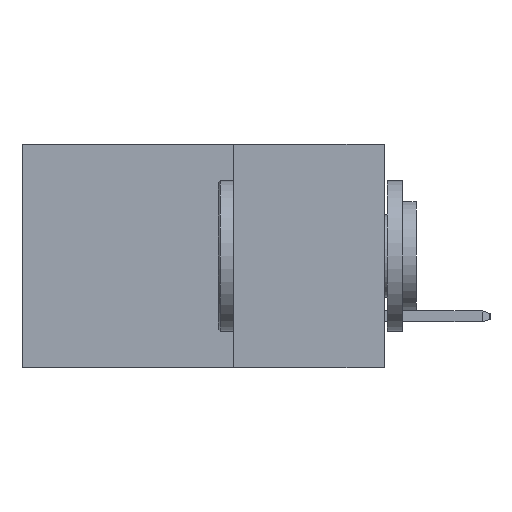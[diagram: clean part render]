
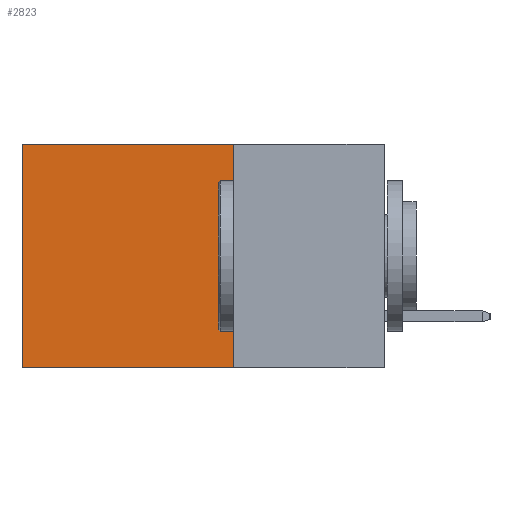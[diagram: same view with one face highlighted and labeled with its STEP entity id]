
A CAD part, left-side view. The second image highlights one B-rep face of the part: STEP entity #2823.
In plain terms, the highlighted planar face has unit normal (-1, 0, 0).
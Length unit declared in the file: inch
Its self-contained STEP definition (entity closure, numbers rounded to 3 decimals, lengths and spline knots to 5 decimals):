
#267 = ORIENTED_EDGE ( 'NONE', *, *, #7602, .F. ) ;
#420 = DIRECTION ( 'NONE',  ( 0., 1., 0. ) ) ;
#733 = VERTEX_POINT ( 'NONE', #10349 ) ;
#1479 = LINE ( 'NONE', #7642, #6083 ) ;
#2122 = CARTESIAN_POINT ( 'NONE',  ( 0.298, 0.25, 0. ) ) ;
#2326 = DIRECTION ( 'NONE',  ( 0., 0., -1. ) ) ;
#2350 = DIRECTION ( 'NONE',  ( 1., 0., 0. ) ) ;
#2458 = VECTOR ( 'NONE', #6980, 39.37008 ) ;
#2641 = ORIENTED_EDGE ( 'NONE', *, *, #8988, .T. ) ;
#2764 = LINE ( 'NONE', #9601, #2458 ) ;
#2819 = FACE_OUTER_BOUND ( 'NONE', #4405, .T. ) ;
#2823 = ADVANCED_FACE ( 'NONE', ( #2819 ), #6957, .F. ) ;
#2941 = CARTESIAN_POINT ( 'NONE',  ( 0.298, 0.25, 0. ) ) ;
#3430 = DIRECTION ( 'NONE',  ( 0., 0., -1. ) ) ;
#4219 = AXIS2_PLACEMENT_3D ( 'NONE', #2122, #2350, #2326 ) ;
#4405 = EDGE_LOOP ( 'NONE', ( #2641, #8296, #267, #8895 ) ) ;
#5016 = VERTEX_POINT ( 'NONE', #10003 ) ;
#5191 = EDGE_CURVE ( 'NONE', #10911, #5016, #8303, .T. ) ;
#5802 = DIRECTION ( 'NONE',  ( 0., 0., -1. ) ) ;
#5884 = VECTOR ( 'NONE', #420, 39.37008 ) ;
#5965 = VERTEX_POINT ( 'NONE', #6104 ) ;
#6083 = VECTOR ( 'NONE', #5802, 39.37008 ) ;
#6104 = CARTESIAN_POINT ( 'NONE',  ( 0.298, 0.25, -0.37 ) ) ;
#6534 = LINE ( 'NONE', #2941, #7092 ) ;
#6957 = PLANE ( 'NONE',  #4219 ) ;
#6980 = DIRECTION ( 'NONE',  ( 0., 1., 0. ) ) ;
#7092 = VECTOR ( 'NONE', #3430, 39.37008 ) ;
#7280 = CARTESIAN_POINT ( 'NONE',  ( 0.298, 0.25, 0. ) ) ;
#7602 = EDGE_CURVE ( 'NONE', #10911, #5965, #6534, .T. ) ;
#7642 = CARTESIAN_POINT ( 'NONE',  ( 0.298, 0.6, 0. ) ) ;
#8296 = ORIENTED_EDGE ( 'NONE', *, *, #11345, .F. ) ;
#8303 = LINE ( 'NONE', #9084, #5884 ) ;
#8895 = ORIENTED_EDGE ( 'NONE', *, *, #5191, .T. ) ;
#8988 = EDGE_CURVE ( 'NONE', #5016, #733, #1479, .T. ) ;
#9084 = CARTESIAN_POINT ( 'NONE',  ( 0.298, 0.25, 0. ) ) ;
#9601 = CARTESIAN_POINT ( 'NONE',  ( 0.298, 0.25, -0.37 ) ) ;
#10003 = CARTESIAN_POINT ( 'NONE',  ( 0.298, 0.6, 0. ) ) ;
#10349 = CARTESIAN_POINT ( 'NONE',  ( 0.298, 0.6, -0.37 ) ) ;
#10911 = VERTEX_POINT ( 'NONE', #7280 ) ;
#11345 = EDGE_CURVE ( 'NONE', #5965, #733, #2764, .T. ) ;
